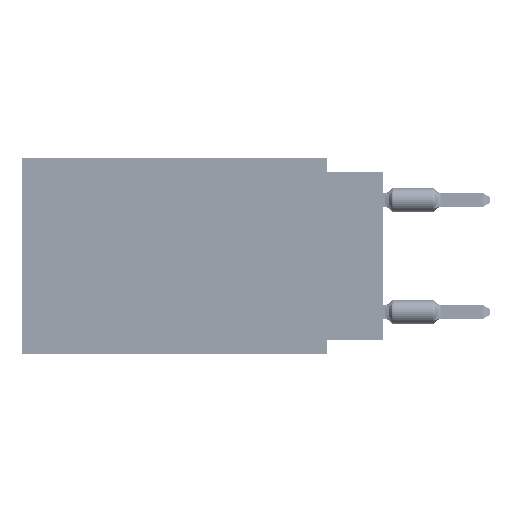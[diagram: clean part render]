
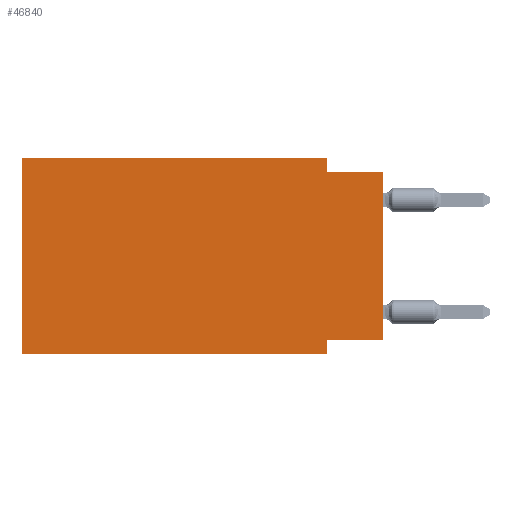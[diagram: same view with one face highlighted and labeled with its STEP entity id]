
A CAD part, left-side view. The second image highlights one B-rep face of the part: STEP entity #46840.
In plain terms, the highlighted planar face has unit normal (-1, 0, 0).
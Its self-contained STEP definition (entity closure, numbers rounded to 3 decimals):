
#1846 = VERTEX_POINT ( 'NONE', #2907 ) ;
#2787 = CARTESIAN_POINT ( 'NONE',  ( 0., 2.54, -0.635 ) ) ;
#2820 = VECTOR ( 'NONE', #58753, 1000. ) ;
#2907 = CARTESIAN_POINT ( 'NONE',  ( 0., 2.54, 0. ) ) ;
#3955 = VERTEX_POINT ( 'NONE', #25812 ) ;
#5190 = CARTESIAN_POINT ( 'NONE',  ( 0., 0., 0. ) ) ;
#5417 = ORIENTED_EDGE ( 'NONE', *, *, #37233, .T. ) ;
#5457 = VECTOR ( 'NONE', #65682, 1000. ) ;
#5744 = CARTESIAN_POINT ( 'NONE',  ( 0., 16.383, 0. ) ) ;
#6694 = VECTOR ( 'NONE', #55147, 1000. ) ;
#7849 = LINE ( 'NONE', #22974, #32358 ) ;
#8716 = DIRECTION ( 'NONE',  ( 0., 1., 0. ) ) ;
#10958 = CARTESIAN_POINT ( 'NONE',  ( 0., 16.383, 0. ) ) ;
#11127 = CARTESIAN_POINT ( 'NONE',  ( 0., 2.54, 0. ) ) ;
#11553 = DIRECTION ( 'NONE',  ( 0., 0., -1. ) ) ;
#12983 = EDGE_CURVE ( 'NONE', #30894, #44443, #71952, .T. ) ;
#13423 = AXIS2_PLACEMENT_3D ( 'NONE', #66730, #86335, #25332 ) ;
#14643 = ORIENTED_EDGE ( 'NONE', *, *, #47854, .F. ) ;
#15560 = ORIENTED_EDGE ( 'NONE', *, *, #47962, .F. ) ;
#17180 = VERTEX_POINT ( 'NONE', #41487 ) ;
#18227 = EDGE_CURVE ( 'NONE', #44443, #1846, #34671, .T. ) ;
#18718 = EDGE_CURVE ( 'NONE', #17180, #39001, #7849, .T. ) ;
#20361 = CARTESIAN_POINT ( 'NONE',  ( 0., 2.54, -8.89 ) ) ;
#22974 = CARTESIAN_POINT ( 'NONE',  ( 0., 0., -8.255 ) ) ;
#25332 = DIRECTION ( 'NONE',  ( 0., 0., -1. ) ) ;
#25812 = CARTESIAN_POINT ( 'NONE',  ( 0., 0., -0.635 ) ) ;
#27041 = VECTOR ( 'NONE', #11553, 1000. ) ;
#29457 = VERTEX_POINT ( 'NONE', #20361 ) ;
#30894 = VERTEX_POINT ( 'NONE', #84943 ) ;
#31403 = LINE ( 'NONE', #74434, #5457 ) ;
#32358 = VECTOR ( 'NONE', #8716, 1000. ) ;
#32619 = CARTESIAN_POINT ( 'NONE',  ( 0., 2.54, -8.89 ) ) ;
#34671 = LINE ( 'NONE', #5744, #6694 ) ;
#34952 = VECTOR ( 'NONE', #38104, 1000. ) ;
#37233 = EDGE_CURVE ( 'NONE', #30894, #29457, #31403, .T. ) ;
#38008 = VECTOR ( 'NONE', #72700, 1000. ) ;
#38104 = DIRECTION ( 'NONE',  ( 0., 0., 1. ) ) ;
#39001 = VERTEX_POINT ( 'NONE', #86446 ) ;
#41487 = CARTESIAN_POINT ( 'NONE',  ( 0., 0., -8.255 ) ) ;
#44443 = VERTEX_POINT ( 'NONE', #50768 ) ;
#44643 = ORIENTED_EDGE ( 'NONE', *, *, #12983, .F. ) ;
#44940 = LINE ( 'NONE', #65873, #2820 ) ;
#45290 = ORIENTED_EDGE ( 'NONE', *, *, #79155, .F. ) ;
#45521 = LINE ( 'NONE', #32619, #38008 ) ;
#46840 = ADVANCED_FACE ( 'NONE', ( #52937 ), #60936, .F. ) ;
#47854 = EDGE_CURVE ( 'NONE', #1846, #77002, #78812, .T. ) ;
#47962 = EDGE_CURVE ( 'NONE', #77002, #3955, #44940, .T. ) ;
#50768 = CARTESIAN_POINT ( 'NONE',  ( 0., 16.383, 0. ) ) ;
#51425 = ORIENTED_EDGE ( 'NONE', *, *, #18227, .F. ) ;
#51954 = ORIENTED_EDGE ( 'NONE', *, *, #18718, .F. ) ;
#52937 = FACE_OUTER_BOUND ( 'NONE', #55200, .T. ) ;
#55147 = DIRECTION ( 'NONE',  ( 0., -1., 0. ) ) ;
#55200 = EDGE_LOOP ( 'NONE', ( #64204, #15560, #14643, #51425, #44643, #5417, #45290, #51954 ) ) ;
#56525 = EDGE_CURVE ( 'NONE', #17180, #3955, #87555, .T. ) ;
#58753 = DIRECTION ( 'NONE',  ( 0., -1., 0. ) ) ;
#59948 = DIRECTION ( 'NONE',  ( 0., 0., 1. ) ) ;
#60936 = PLANE ( 'NONE',  #13423 ) ;
#64204 = ORIENTED_EDGE ( 'NONE', *, *, #56525, .T. ) ;
#64931 = VECTOR ( 'NONE', #59948, 1000. ) ;
#65682 = DIRECTION ( 'NONE',  ( 0., -1., 0. ) ) ;
#65873 = CARTESIAN_POINT ( 'NONE',  ( 0., 0., -0.635 ) ) ;
#66730 = CARTESIAN_POINT ( 'NONE',  ( 0., 16.383, 0. ) ) ;
#71952 = LINE ( 'NONE', #10958, #34952 ) ;
#72700 = DIRECTION ( 'NONE',  ( 0., 0., -1. ) ) ;
#74434 = CARTESIAN_POINT ( 'NONE',  ( 0., 16.383, -8.89 ) ) ;
#77002 = VERTEX_POINT ( 'NONE', #2787 ) ;
#78812 = LINE ( 'NONE', #11127, #27041 ) ;
#79155 = EDGE_CURVE ( 'NONE', #39001, #29457, #45521, .T. ) ;
#84943 = CARTESIAN_POINT ( 'NONE',  ( 0., 16.383, -8.89 ) ) ;
#86335 = DIRECTION ( 'NONE',  ( 1., 0., 0. ) ) ;
#86446 = CARTESIAN_POINT ( 'NONE',  ( 0., 2.54, -8.255 ) ) ;
#87555 = LINE ( 'NONE', #5190, #64931 ) ;
